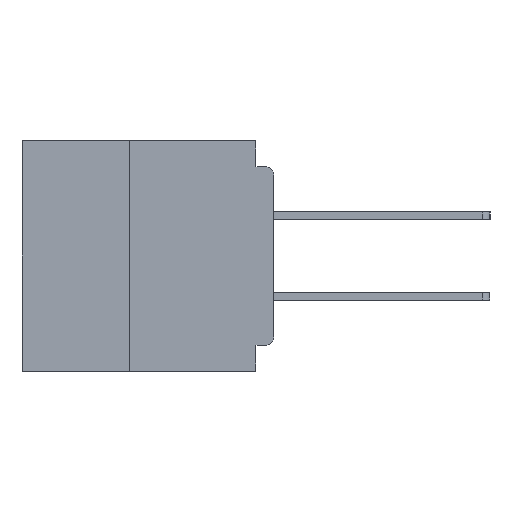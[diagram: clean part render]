
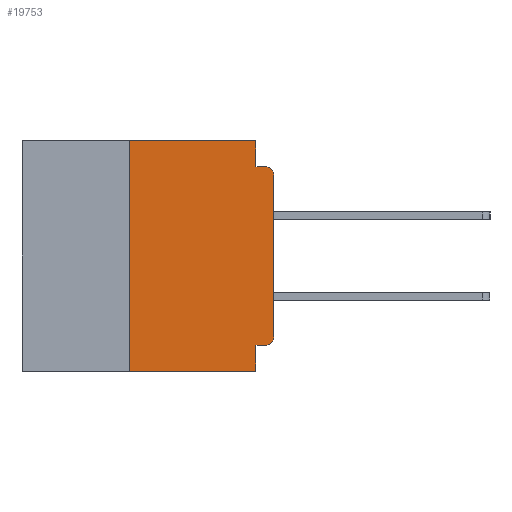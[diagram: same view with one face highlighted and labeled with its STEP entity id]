
A CAD part, left-side view. The second image highlights one B-rep face of the part: STEP entity #19753.
In plain terms, the highlighted planar face has unit normal (-1, 0, 0).
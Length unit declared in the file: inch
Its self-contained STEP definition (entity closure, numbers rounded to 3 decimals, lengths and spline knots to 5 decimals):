
#220 = DIRECTION ( 'NONE',  ( 0., 0., 1. ) ) ;
#928 = VERTEX_POINT ( 'NONE', #35446 ) ;
#971 = VERTEX_POINT ( 'NONE', #8191 ) ;
#1024 = VERTEX_POINT ( 'NONE', #1781 ) ;
#1467 = DIRECTION ( 'NONE',  ( 0., 0., -1. ) ) ;
#1781 = CARTESIAN_POINT ( 'NONE',  ( 0., 0.25, 0. ) ) ;
#2708 = CARTESIAN_POINT ( 'NONE',  ( 0., 0., -0.34 ) ) ;
#2892 = EDGE_CURVE ( 'NONE', #6599, #1024, #21522, .T. ) ;
#4522 = ORIENTED_EDGE ( 'NONE', *, *, #23025, .T. ) ;
#4667 = ORIENTED_EDGE ( 'NONE', *, *, #26413, .T. ) ;
#4980 = CARTESIAN_POINT ( 'NONE',  ( 0., 0.031, 0. ) ) ;
#5041 = LINE ( 'NONE', #22967, #27025 ) ;
#5060 = DIRECTION ( 'NONE',  ( 0., -1., 0. ) ) ;
#5244 = ORIENTED_EDGE ( 'NONE', *, *, #13978, .F. ) ;
#5645 = CARTESIAN_POINT ( 'NONE',  ( 0., 0.031, -0.4 ) ) ;
#5896 = ORIENTED_EDGE ( 'NONE', *, *, #11210, .F. ) ;
#6440 = ORIENTED_EDGE ( 'NONE', *, *, #18374, .F. ) ;
#6599 = VERTEX_POINT ( 'NONE', #12198 ) ;
#6602 = CARTESIAN_POINT ( 'NONE',  ( 0., 0., -0.355 ) ) ;
#6841 = AXIS2_PLACEMENT_3D ( 'NONE', #17176, #8464, #28532 ) ;
#7287 = EDGE_LOOP ( 'NONE', ( #4667, #4522, #5244, #6440, #5896, #7689, #7584, #7452, #8407, #10411 ) ) ;
#7452 = ORIENTED_EDGE ( 'NONE', *, *, #12307, .F. ) ;
#7584 = ORIENTED_EDGE ( 'NONE', *, *, #12950, .T. ) ;
#7689 = ORIENTED_EDGE ( 'NONE', *, *, #2892, .F. ) ;
#8130 = EDGE_CURVE ( 'NONE', #18575, #15893, #23284, .T. ) ;
#8191 = CARTESIAN_POINT ( 'NONE',  ( 0., 0., -0.06 ) ) ;
#8407 = ORIENTED_EDGE ( 'NONE', *, *, #22925, .F. ) ;
#8464 = DIRECTION ( 'NONE',  ( 1., 0., 0. ) ) ;
#8651 = AXIS2_PLACEMENT_3D ( 'NONE', #35555, #18851, #1467 ) ;
#10411 = ORIENTED_EDGE ( 'NONE', *, *, #8130, .T. ) ;
#10434 = CARTESIAN_POINT ( 'NONE',  ( 0., 0.031, -0.4 ) ) ;
#11210 = EDGE_CURVE ( 'NONE', #1024, #34376, #5041, .T. ) ;
#12000 = CARTESIAN_POINT ( 'NONE',  ( 0., 0.031, 0. ) ) ;
#12198 = CARTESIAN_POINT ( 'NONE',  ( 0., 0.25, -0.4 ) ) ;
#12307 = EDGE_CURVE ( 'NONE', #30439, #31467, #18837, .T. ) ;
#12950 = EDGE_CURVE ( 'NONE', #6599, #31467, #26686, .T. ) ;
#13854 = AXIS2_PLACEMENT_3D ( 'NONE', #31033, #14012, #33822 ) ;
#13978 = EDGE_CURVE ( 'NONE', #19333, #928, #31447, .T. ) ;
#14012 = DIRECTION ( 'NONE',  ( -1., 0., 0. ) ) ;
#15893 = VERTEX_POINT ( 'NONE', #2708 ) ;
#16757 = LINE ( 'NONE', #4980, #22544 ) ;
#16782 = CARTESIAN_POINT ( 'NONE',  ( 0., 0., -0.045 ) ) ;
#17176 = CARTESIAN_POINT ( 'NONE',  ( 0., 0.437, 0. ) ) ;
#17642 = CARTESIAN_POINT ( 'NONE',  ( 0., 0., 0. ) ) ;
#17943 = VECTOR ( 'NONE', #27673, 39.37008 ) ;
#18374 = EDGE_CURVE ( 'NONE', #34376, #19333, #16757, .T. ) ;
#18575 = VERTEX_POINT ( 'NONE', #25952 ) ;
#18837 = LINE ( 'NONE', #10434, #17943 ) ;
#18851 = DIRECTION ( 'NONE',  ( -1., 0., 0. ) ) ;
#19333 = VERTEX_POINT ( 'NONE', #32080 ) ;
#19753 = ADVANCED_FACE ( 'NONE', ( #29506 ), #33975, .F. ) ;
#20664 = VECTOR ( 'NONE', #30286, 39.37008 ) ;
#21057 = DIRECTION ( 'NONE',  ( 0., 1., 0. ) ) ;
#21420 = VECTOR ( 'NONE', #220, 39.37008 ) ;
#21522 = LINE ( 'NONE', #26074, #20664 ) ;
#22544 = VECTOR ( 'NONE', #30748, 39.37008 ) ;
#22925 = EDGE_CURVE ( 'NONE', #18575, #30439, #29648, .T. ) ;
#22967 = CARTESIAN_POINT ( 'NONE',  ( 0., 0.437, 0. ) ) ;
#23025 = EDGE_CURVE ( 'NONE', #971, #928, #35237, .T. ) ;
#23284 = CIRCLE ( 'NONE', #13854, 0.015 ) ;
#25299 = DIRECTION ( 'NONE',  ( 0., -1., 0. ) ) ;
#25952 = CARTESIAN_POINT ( 'NONE',  ( 0., 0.015, -0.355 ) ) ;
#26074 = CARTESIAN_POINT ( 'NONE',  ( 0., 0.25, -0.4 ) ) ;
#26413 = EDGE_CURVE ( 'NONE', #15893, #971, #34542, .T. ) ;
#26686 = LINE ( 'NONE', #28021, #33247 ) ;
#27025 = VECTOR ( 'NONE', #28622, 39.37008 ) ;
#27673 = DIRECTION ( 'NONE',  ( 0., 0., -1. ) ) ;
#28021 = CARTESIAN_POINT ( 'NONE',  ( 0., 0.437, -0.4 ) ) ;
#28532 = DIRECTION ( 'NONE',  ( 0., 0., -1. ) ) ;
#28622 = DIRECTION ( 'NONE',  ( 0., -1., 0. ) ) ;
#28783 = CARTESIAN_POINT ( 'NONE',  ( 0., 0.031, -0.355 ) ) ;
#28798 = VECTOR ( 'NONE', #21057, 39.37008 ) ;
#29506 = FACE_OUTER_BOUND ( 'NONE', #7287, .T. ) ;
#29648 = LINE ( 'NONE', #6602, #28798 ) ;
#30286 = DIRECTION ( 'NONE',  ( 0., 0., 1. ) ) ;
#30439 = VERTEX_POINT ( 'NONE', #28783 ) ;
#30748 = DIRECTION ( 'NONE',  ( 0., 0., -1. ) ) ;
#31033 = CARTESIAN_POINT ( 'NONE',  ( 0., 0.015, -0.34 ) ) ;
#31447 = LINE ( 'NONE', #16782, #36136 ) ;
#31467 = VERTEX_POINT ( 'NONE', #5645 ) ;
#32080 = CARTESIAN_POINT ( 'NONE',  ( 0., 0.031, -0.045 ) ) ;
#33247 = VECTOR ( 'NONE', #25299, 39.37008 ) ;
#33822 = DIRECTION ( 'NONE',  ( 0., 0., -1. ) ) ;
#33975 = PLANE ( 'NONE',  #6841 ) ;
#34376 = VERTEX_POINT ( 'NONE', #12000 ) ;
#34542 = LINE ( 'NONE', #17642, #21420 ) ;
#35237 = CIRCLE ( 'NONE', #8651, 0.015 ) ;
#35446 = CARTESIAN_POINT ( 'NONE',  ( 0., 0.015, -0.045 ) ) ;
#35555 = CARTESIAN_POINT ( 'NONE',  ( 0., 0.015, -0.06 ) ) ;
#36136 = VECTOR ( 'NONE', #5060, 39.37008 ) ;
